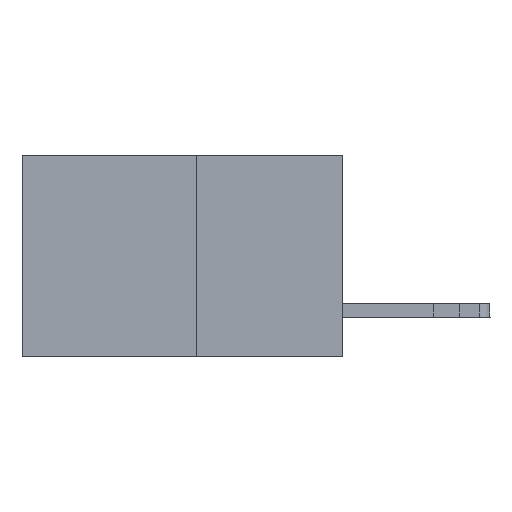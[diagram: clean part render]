
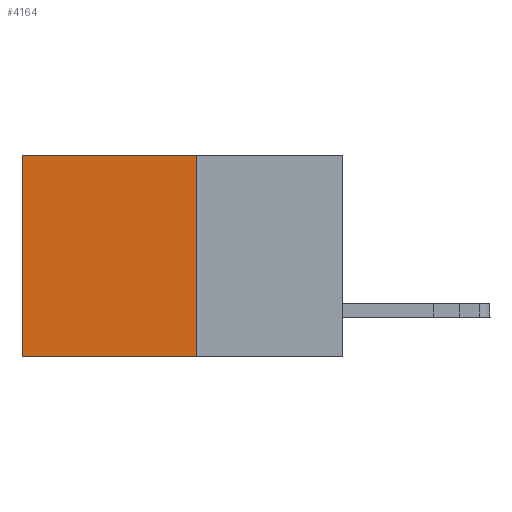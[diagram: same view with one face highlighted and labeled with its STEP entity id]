
A CAD part, left-side view. The second image highlights one B-rep face of the part: STEP entity #4164.
In plain terms, the highlighted planar face has unit normal (-1, 0, 0).
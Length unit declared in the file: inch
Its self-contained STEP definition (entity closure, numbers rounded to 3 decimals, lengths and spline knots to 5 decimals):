
#535 = VECTOR ( 'NONE', #8946, 39.37008 ) ;
#1819 = DIRECTION ( 'NONE',  ( 0., 0., -1. ) ) ;
#1823 = DIRECTION ( 'NONE',  ( 1., 0., 0. ) ) ;
#1861 = PLANE ( 'NONE',  #2588 ) ;
#2011 = EDGE_CURVE ( 'NONE', #6225, #8373, #3057, .T. ) ;
#2155 = CARTESIAN_POINT ( 'NONE',  ( 0.277, 0.27, -0.37 ) ) ;
#2262 = VECTOR ( 'NONE', #5307, 39.37008 ) ;
#2588 = AXIS2_PLACEMENT_3D ( 'NONE', #2155, #1823, #1819 ) ;
#3057 = LINE ( 'NONE', #10916, #6325 ) ;
#3770 = LINE ( 'NONE', #13703, #535 ) ;
#4164 = ADVANCED_FACE ( 'NONE', ( #7215 ), #1861, .F. ) ;
#4274 = CARTESIAN_POINT ( 'NONE',  ( 0.277, 0.27, 0. ) ) ;
#4838 = VECTOR ( 'NONE', #10392, 39.37008 ) ;
#5307 = DIRECTION ( 'NONE',  ( 0., 0., -1. ) ) ;
#5810 = ORIENTED_EDGE ( 'NONE', *, *, #2011, .F. ) ;
#6225 = VERTEX_POINT ( 'NONE', #7240 ) ;
#6325 = VECTOR ( 'NONE', #13161, 39.37008 ) ;
#6665 = CARTESIAN_POINT ( 'NONE',  ( 0.277, 0.59, -0.37 ) ) ;
#7129 = ORIENTED_EDGE ( 'NONE', *, *, #10547, .F. ) ;
#7215 = FACE_OUTER_BOUND ( 'NONE', #11601, .T. ) ;
#7240 = CARTESIAN_POINT ( 'NONE',  ( 0.277, 0.27, -0.37 ) ) ;
#7878 = VERTEX_POINT ( 'NONE', #11847 ) ;
#8217 = ORIENTED_EDGE ( 'NONE', *, *, #10843, .T. ) ;
#8373 = VERTEX_POINT ( 'NONE', #6665 ) ;
#8946 = DIRECTION ( 'NONE',  ( 0., 0., -1. ) ) ;
#9172 = CARTESIAN_POINT ( 'NONE',  ( 0.277, 0.27, 0. ) ) ;
#10392 = DIRECTION ( 'NONE',  ( 0., 1., 0. ) ) ;
#10547 = EDGE_CURVE ( 'NONE', #12409, #6225, #15014, .T. ) ;
#10843 = EDGE_CURVE ( 'NONE', #7878, #8373, #3770, .T. ) ;
#10916 = CARTESIAN_POINT ( 'NONE',  ( 0.277, 0.27, -0.37 ) ) ;
#11601 = EDGE_LOOP ( 'NONE', ( #8217, #5810, #7129, #13211 ) ) ;
#11847 = CARTESIAN_POINT ( 'NONE',  ( 0.277, 0.59, 0. ) ) ;
#12409 = VERTEX_POINT ( 'NONE', #4274 ) ;
#12584 = CARTESIAN_POINT ( 'NONE',  ( 0.277, 0.27, -0.37 ) ) ;
#13161 = DIRECTION ( 'NONE',  ( 0., 1., 0. ) ) ;
#13211 = ORIENTED_EDGE ( 'NONE', *, *, #15114, .T. ) ;
#13703 = CARTESIAN_POINT ( 'NONE',  ( 0.277, 0.59, -0.37 ) ) ;
#15014 = LINE ( 'NONE', #12584, #2262 ) ;
#15091 = LINE ( 'NONE', #9172, #4838 ) ;
#15114 = EDGE_CURVE ( 'NONE', #12409, #7878, #15091, .T. ) ;
